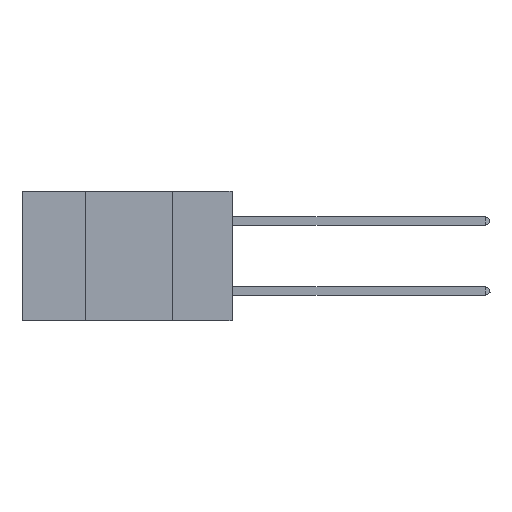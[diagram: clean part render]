
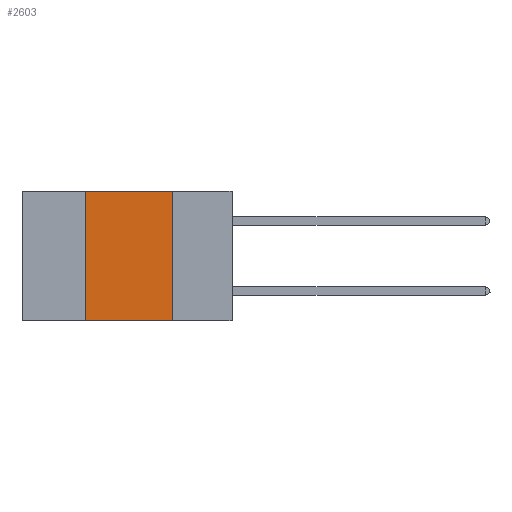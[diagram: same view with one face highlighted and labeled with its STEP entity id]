
A CAD part, left-side view. The second image highlights one B-rep face of the part: STEP entity #2603.
In plain terms, the highlighted planar face has unit normal (-1, 0, 0).
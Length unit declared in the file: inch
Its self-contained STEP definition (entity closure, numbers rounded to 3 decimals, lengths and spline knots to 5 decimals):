
#17 = VECTOR ( 'NONE', #5211, 39.37008 ) ;
#459 = PLANE ( 'NONE',  #11794 ) ;
#515 = CARTESIAN_POINT ( 'NONE',  ( 0., 0.6, -0.37 ) ) ;
#853 = VERTEX_POINT ( 'NONE', #20475 ) ;
#2258 = EDGE_CURVE ( 'NONE', #8569, #10898, #15645, .T. ) ;
#2559 = CARTESIAN_POINT ( 'NONE',  ( 0., 0.6, 0. ) ) ;
#2603 = ADVANCED_FACE ( 'NONE', ( #19396 ), #459, .F. ) ;
#2995 = ORIENTED_EDGE ( 'NONE', *, *, #8634, .F. ) ;
#3025 = EDGE_CURVE ( 'NONE', #853, #23327, #5914, .T. ) ;
#4505 = DIRECTION ( 'NONE',  ( 1., 0., 0. ) ) ;
#5211 = DIRECTION ( 'NONE',  ( 0., -1., 0. ) ) ;
#5914 = LINE ( 'NONE', #25662, #13134 ) ;
#6649 = DIRECTION ( 'NONE',  ( 0., 0., -1. ) ) ;
#7924 = DIRECTION ( 'NONE',  ( 0., 0., 1. ) ) ;
#8116 = LINE ( 'NONE', #515, #12826 ) ;
#8569 = VERTEX_POINT ( 'NONE', #23059 ) ;
#8634 = EDGE_CURVE ( 'NONE', #10898, #853, #18193, .T. ) ;
#10600 = DIRECTION ( 'NONE',  ( 0., -1., 0. ) ) ;
#10898 = VERTEX_POINT ( 'NONE', #20641 ) ;
#11641 = CARTESIAN_POINT ( 'NONE',  ( 0., 0.17, -0.37 ) ) ;
#11794 = AXIS2_PLACEMENT_3D ( 'NONE', #2559, #4505, #18514 ) ;
#12826 = VECTOR ( 'NONE', #10600, 39.37008 ) ;
#13134 = VECTOR ( 'NONE', #6649, 39.37008 ) ;
#13557 = ORIENTED_EDGE ( 'NONE', *, *, #2258, .F. ) ;
#13890 = EDGE_LOOP ( 'NONE', ( #18311, #2995, #13557, #23060 ) ) ;
#14865 = EDGE_CURVE ( 'NONE', #8569, #23327, #8116, .T. ) ;
#15645 = LINE ( 'NONE', #19213, #19095 ) ;
#18193 = LINE ( 'NONE', #19296, #17 ) ;
#18311 = ORIENTED_EDGE ( 'NONE', *, *, #3025, .F. ) ;
#18514 = DIRECTION ( 'NONE',  ( 0., 0., -1. ) ) ;
#19095 = VECTOR ( 'NONE', #7924, 39.37008 ) ;
#19213 = CARTESIAN_POINT ( 'NONE',  ( 0., 0.42, 0. ) ) ;
#19296 = CARTESIAN_POINT ( 'NONE',  ( 0., 0.6, 0. ) ) ;
#19396 = FACE_OUTER_BOUND ( 'NONE', #13890, .T. ) ;
#20475 = CARTESIAN_POINT ( 'NONE',  ( 0., 0.17, 0. ) ) ;
#20641 = CARTESIAN_POINT ( 'NONE',  ( 0., 0.42, 0. ) ) ;
#23059 = CARTESIAN_POINT ( 'NONE',  ( 0., 0.42, -0.37 ) ) ;
#23060 = ORIENTED_EDGE ( 'NONE', *, *, #14865, .T. ) ;
#23327 = VERTEX_POINT ( 'NONE', #11641 ) ;
#25662 = CARTESIAN_POINT ( 'NONE',  ( 0., 0.17, 0. ) ) ;
